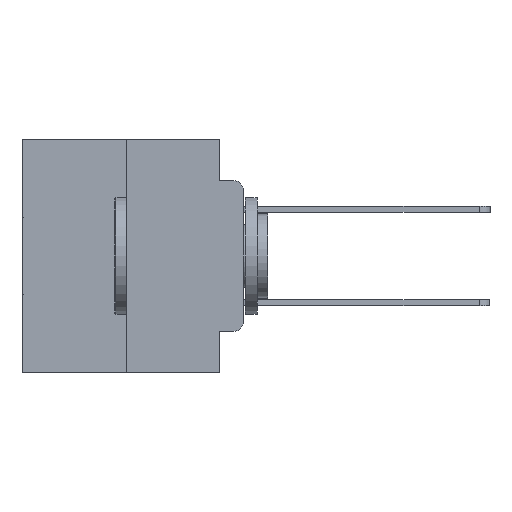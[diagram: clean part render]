
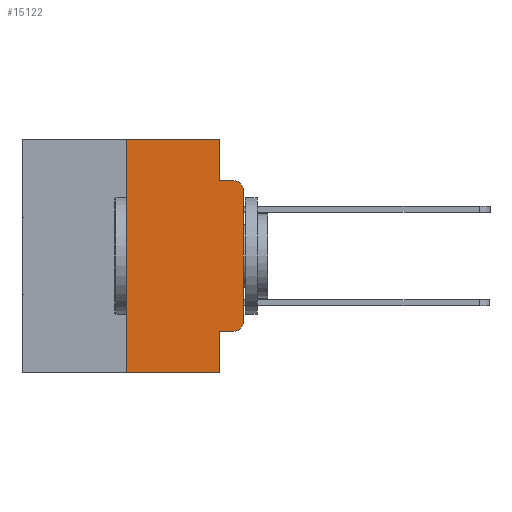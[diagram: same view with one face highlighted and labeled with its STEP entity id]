
A CAD part, left-side view. The second image highlights one B-rep face of the part: STEP entity #15122.
In plain terms, the highlighted planar face has unit normal (-1, 0, 0).
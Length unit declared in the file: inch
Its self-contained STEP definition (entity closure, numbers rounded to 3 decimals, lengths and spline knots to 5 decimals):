
#144 = VERTEX_POINT ( 'NONE', #18385 ) ;
#188 = VERTEX_POINT ( 'NONE', #27417 ) ;
#329 = DIRECTION ( 'NONE',  ( 0., 0., 1. ) ) ;
#1000 = DIRECTION ( 'NONE',  ( -1., 0., 0. ) ) ;
#2076 = DIRECTION ( 'NONE',  ( 0., 0., -1. ) ) ;
#2176 = VECTOR ( 'NONE', #12660, 39.37008 ) ;
#2665 = VERTEX_POINT ( 'NONE', #11607 ) ;
#3241 = CARTESIAN_POINT ( 'NONE',  ( 0., 0.473, 0. ) ) ;
#3242 = LINE ( 'NONE', #14172, #26615 ) ;
#3312 = CARTESIAN_POINT ( 'NONE',  ( 0., 0.051, 0. ) ) ;
#3854 = ORIENTED_EDGE ( 'NONE', *, *, #7673, .T. ) ;
#4179 = CARTESIAN_POINT ( 'NONE',  ( 0., 0., -0.3915 ) ) ;
#4375 = VECTOR ( 'NONE', #29381, 39.37008 ) ;
#5008 = CARTESIAN_POINT ( 'NONE',  ( 0., 0.051, -0.4115 ) ) ;
#5218 = PLANE ( 'NONE',  #16956 ) ;
#5328 = VECTOR ( 'NONE', #21680, 39.37008 ) ;
#6437 = AXIS2_PLACEMENT_3D ( 'NONE', #29973, #16204, #2076 ) ;
#7673 = EDGE_CURVE ( 'NONE', #18951, #22395, #12352, .T. ) ;
#8670 = ORIENTED_EDGE ( 'NONE', *, *, #12381, .F. ) ;
#9066 = LINE ( 'NONE', #11672, #27578 ) ;
#9256 = EDGE_CURVE ( 'NONE', #9822, #18951, #12300, .T. ) ;
#9822 = VERTEX_POINT ( 'NONE', #5008 ) ;
#9960 = DIRECTION ( 'NONE',  ( 0., 0., -1. ) ) ;
#10279 = DIRECTION ( 'NONE',  ( 0., -1., 0. ) ) ;
#10902 = VERTEX_POINT ( 'NONE', #29986 ) ;
#11209 = ORIENTED_EDGE ( 'NONE', *, *, #21736, .T. ) ;
#11607 = CARTESIAN_POINT ( 'NONE',  ( 0., 0., -0.1085 ) ) ;
#11672 = CARTESIAN_POINT ( 'NONE',  ( 0., 0.051, 0. ) ) ;
#12300 = LINE ( 'NONE', #14631, #5328 ) ;
#12352 = CIRCLE ( 'NONE', #6437, 0.02 ) ;
#12381 = EDGE_CURVE ( 'NONE', #9822, #144, #14699, .T. ) ;
#12654 = ORIENTED_EDGE ( 'NONE', *, *, #15491, .F. ) ;
#12660 = DIRECTION ( 'NONE',  ( 0., 0., -1. ) ) ;
#13377 = ORIENTED_EDGE ( 'NONE', *, *, #17115, .F. ) ;
#13910 = EDGE_CURVE ( 'NONE', #19418, #10902, #3242, .T. ) ;
#14080 = ORIENTED_EDGE ( 'NONE', *, *, #23107, .T. ) ;
#14172 = CARTESIAN_POINT ( 'NONE',  ( 0., 0.25, 0. ) ) ;
#14631 = CARTESIAN_POINT ( 'NONE',  ( 0., 0.051, -0.4115 ) ) ;
#14699 = LINE ( 'NONE', #3312, #2176 ) ;
#14820 = ORIENTED_EDGE ( 'NONE', *, *, #9256, .T. ) ;
#15122 = ADVANCED_FACE ( 'NONE', ( #25454 ), #5218, .F. ) ;
#15154 = CARTESIAN_POINT ( 'NONE',  ( 0., 0.02, -0.1085 ) ) ;
#15491 = EDGE_CURVE ( 'NONE', #188, #18036, #9066, .T. ) ;
#15940 = LINE ( 'NONE', #21857, #22126 ) ;
#16204 = DIRECTION ( 'NONE',  ( -1., 0., 0. ) ) ;
#16558 = DIRECTION ( 'NONE',  ( 0., 0., 1. ) ) ;
#16666 = ORIENTED_EDGE ( 'NONE', *, *, #26401, .T. ) ;
#16834 = LINE ( 'NONE', #22926, #4375 ) ;
#16956 = AXIS2_PLACEMENT_3D ( 'NONE', #21546, #23884, #9960 ) ;
#17075 = EDGE_CURVE ( 'NONE', #18036, #29873, #15940, .T. ) ;
#17115 = EDGE_CURVE ( 'NONE', #10902, #188, #21377, .T. ) ;
#17537 = DIRECTION ( 'NONE',  ( 0., 0., -1. ) ) ;
#18036 = VERTEX_POINT ( 'NONE', #18624 ) ;
#18385 = CARTESIAN_POINT ( 'NONE',  ( 0., 0.051, -0.5 ) ) ;
#18624 = CARTESIAN_POINT ( 'NONE',  ( 0., 0.051, -0.0885 ) ) ;
#18662 = AXIS2_PLACEMENT_3D ( 'NONE', #15154, #1000, #17537 ) ;
#18841 = CARTESIAN_POINT ( 'NONE',  ( 0., 0.25, -0.5 ) ) ;
#18951 = VERTEX_POINT ( 'NONE', #24247 ) ;
#19137 = VECTOR ( 'NONE', #329, 39.37008 ) ;
#19418 = VERTEX_POINT ( 'NONE', #18841 ) ;
#19450 = CIRCLE ( 'NONE', #18662, 0.02 ) ;
#19896 = EDGE_LOOP ( 'NONE', ( #16666, #11209, #23564, #12654, #13377, #25748, #14080, #8670, #14820, #3854 ) ) ;
#20656 = VECTOR ( 'NONE', #28895, 39.37008 ) ;
#21377 = LINE ( 'NONE', #3241, #20656 ) ;
#21546 = CARTESIAN_POINT ( 'NONE',  ( 0., 0.473, 0. ) ) ;
#21680 = DIRECTION ( 'NONE',  ( 0., -1., 0. ) ) ;
#21696 = CARTESIAN_POINT ( 'NONE',  ( 0., 0.02, -0.0885 ) ) ;
#21736 = EDGE_CURVE ( 'NONE', #2665, #29873, #19450, .T. ) ;
#21857 = CARTESIAN_POINT ( 'NONE',  ( 0., 0.051, -0.0885 ) ) ;
#22126 = VECTOR ( 'NONE', #10279, 39.37008 ) ;
#22395 = VERTEX_POINT ( 'NONE', #4179 ) ;
#22926 = CARTESIAN_POINT ( 'NONE',  ( 0., 0.473, -0.5 ) ) ;
#23107 = EDGE_CURVE ( 'NONE', #19418, #144, #16834, .T. ) ;
#23564 = ORIENTED_EDGE ( 'NONE', *, *, #17075, .F. ) ;
#23884 = DIRECTION ( 'NONE',  ( 1., 0., 0. ) ) ;
#24247 = CARTESIAN_POINT ( 'NONE',  ( 0., 0.02, -0.4115 ) ) ;
#25454 = FACE_OUTER_BOUND ( 'NONE', #19896, .T. ) ;
#25748 = ORIENTED_EDGE ( 'NONE', *, *, #13910, .F. ) ;
#26150 = CARTESIAN_POINT ( 'NONE',  ( 0., 0., 0. ) ) ;
#26401 = EDGE_CURVE ( 'NONE', #22395, #2665, #26747, .T. ) ;
#26615 = VECTOR ( 'NONE', #16558, 39.37008 ) ;
#26747 = LINE ( 'NONE', #26150, #19137 ) ;
#27417 = CARTESIAN_POINT ( 'NONE',  ( 0., 0.051, 0. ) ) ;
#27578 = VECTOR ( 'NONE', #30126, 39.37008 ) ;
#28895 = DIRECTION ( 'NONE',  ( 0., -1., 0. ) ) ;
#29381 = DIRECTION ( 'NONE',  ( 0., -1., 0. ) ) ;
#29873 = VERTEX_POINT ( 'NONE', #21696 ) ;
#29973 = CARTESIAN_POINT ( 'NONE',  ( 0., 0.02, -0.3915 ) ) ;
#29986 = CARTESIAN_POINT ( 'NONE',  ( 0., 0.25, 0. ) ) ;
#30126 = DIRECTION ( 'NONE',  ( 0., 0., -1. ) ) ;
